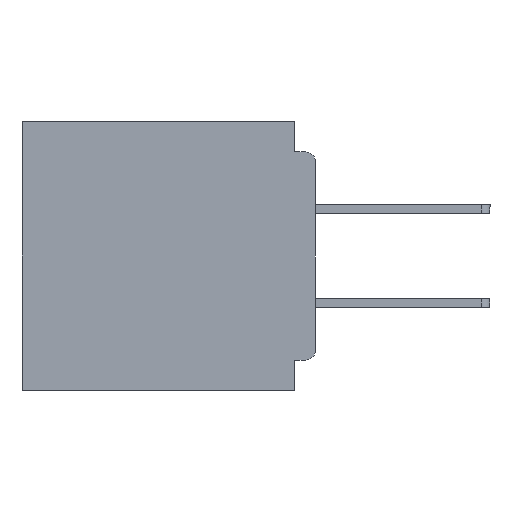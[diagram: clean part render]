
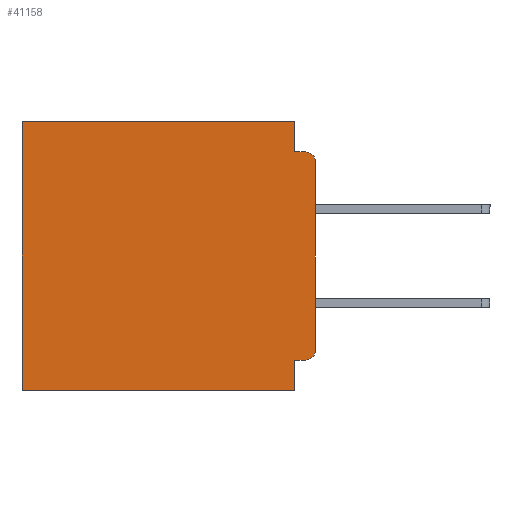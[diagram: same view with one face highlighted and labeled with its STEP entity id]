
A CAD part, left-side view. The second image highlights one B-rep face of the part: STEP entity #41158.
In plain terms, the highlighted planar face has unit normal (-1, 0, 0).
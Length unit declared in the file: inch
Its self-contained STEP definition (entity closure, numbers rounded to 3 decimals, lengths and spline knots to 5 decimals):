
#949 = EDGE_CURVE ( 'NONE', #23694, #44649, #47335, .T. ) ;
#1743 = VERTEX_POINT ( 'NONE', #13248 ) ;
#1891 = ORIENTED_EDGE ( 'NONE', *, *, #44778, .F. ) ;
#1966 = DIRECTION ( 'NONE',  ( 0., 0., -1. ) ) ;
#2060 = EDGE_CURVE ( 'NONE', #1743, #26895, #12864, .T. ) ;
#2621 = LINE ( 'NONE', #42442, #40899 ) ;
#3561 = ORIENTED_EDGE ( 'NONE', *, *, #24963, .F. ) ;
#4515 = LINE ( 'NONE', #44449, #32737 ) ;
#5194 = VECTOR ( 'NONE', #18913, 39.37008 ) ;
#5952 = CARTESIAN_POINT ( 'NONE',  ( 0.3, 0.015, -0.06 ) ) ;
#6795 = CARTESIAN_POINT ( 'NONE',  ( 0.3, 0.437, 0. ) ) ;
#7148 = LINE ( 'NONE', #17382, #15026 ) ;
#7255 = EDGE_CURVE ( 'NONE', #13311, #23694, #4515, .T. ) ;
#7734 = CARTESIAN_POINT ( 'NONE',  ( 0.3, 0.015, -0.34 ) ) ;
#9038 = VERTEX_POINT ( 'NONE', #13442 ) ;
#9049 = EDGE_CURVE ( 'NONE', #20914, #44649, #18894, .T. ) ;
#9212 = LINE ( 'NONE', #17850, #28392 ) ;
#9858 = DIRECTION ( 'NONE',  ( 0., 0., -1. ) ) ;
#9873 = AXIS2_PLACEMENT_3D ( 'NONE', #5952, #32758, #9858 ) ;
#10303 = CARTESIAN_POINT ( 'NONE',  ( 0.3, 0.015, -0.045 ) ) ;
#10361 = DIRECTION ( 'NONE',  ( 0., 0., -1. ) ) ;
#10564 = CARTESIAN_POINT ( 'NONE',  ( 0.3, 0., -0.06 ) ) ;
#10744 = DIRECTION ( 'NONE',  ( 1., 0., 0. ) ) ;
#11094 = ORIENTED_EDGE ( 'NONE', *, *, #7255, .F. ) ;
#11638 = DIRECTION ( 'NONE',  ( 0., 0., -1. ) ) ;
#11641 = VECTOR ( 'NONE', #14758, 39.37008 ) ;
#12192 = ORIENTED_EDGE ( 'NONE', *, *, #46642, .T. ) ;
#12536 = VERTEX_POINT ( 'NONE', #6795 ) ;
#12864 = LINE ( 'NONE', #44875, #11641 ) ;
#13248 = CARTESIAN_POINT ( 'NONE',  ( 0.3, 0.031, -0.355 ) ) ;
#13311 = VERTEX_POINT ( 'NONE', #25692 ) ;
#13442 = CARTESIAN_POINT ( 'NONE',  ( 0.3, 0.015, -0.355 ) ) ;
#13733 = EDGE_CURVE ( 'NONE', #12536, #34323, #7148, .T. ) ;
#14758 = DIRECTION ( 'NONE',  ( 0., 0., -1. ) ) ;
#15026 = VECTOR ( 'NONE', #1966, 39.37008 ) ;
#15034 = CARTESIAN_POINT ( 'NONE',  ( 0.3, 0., -0.355 ) ) ;
#17126 = VECTOR ( 'NONE', #33660, 39.37008 ) ;
#17382 = CARTESIAN_POINT ( 'NONE',  ( 0.3, 0.437, -0.4 ) ) ;
#17461 = LINE ( 'NONE', #19959, #38786 ) ;
#17728 = ORIENTED_EDGE ( 'NONE', *, *, #9049, .T. ) ;
#17850 = CARTESIAN_POINT ( 'NONE',  ( 0.3, 0., -0.4 ) ) ;
#18521 = CARTESIAN_POINT ( 'NONE',  ( 0.3, 0., -0.4 ) ) ;
#18894 = CIRCLE ( 'NONE', #9873, 0.015 ) ;
#18913 = DIRECTION ( 'NONE',  ( 0., 1., 0. ) ) ;
#19959 = CARTESIAN_POINT ( 'NONE',  ( 0.3, 0., -0.4 ) ) ;
#20795 = EDGE_LOOP ( 'NONE', ( #25402, #17728, #23569, #11094, #36099, #27829, #3561, #35887, #1891, #12192 ) ) ;
#20914 = VERTEX_POINT ( 'NONE', #10564 ) ;
#22131 = EDGE_CURVE ( 'NONE', #13311, #12536, #2621, .T. ) ;
#23569 = ORIENTED_EDGE ( 'NONE', *, *, #949, .F. ) ;
#23694 = VERTEX_POINT ( 'NONE', #44800 ) ;
#24091 = CARTESIAN_POINT ( 'NONE',  ( 0.3, 0.031, -0.4 ) ) ;
#24963 = EDGE_CURVE ( 'NONE', #26895, #34323, #17461, .T. ) ;
#25402 = ORIENTED_EDGE ( 'NONE', *, *, #41027, .F. ) ;
#25692 = CARTESIAN_POINT ( 'NONE',  ( 0.3, 0.031, 0. ) ) ;
#26142 = DIRECTION ( 'NONE',  ( 0., 0., -1. ) ) ;
#26178 = CARTESIAN_POINT ( 'NONE',  ( 0.3, 0., -0.045 ) ) ;
#26895 = VERTEX_POINT ( 'NONE', #24091 ) ;
#27051 = VERTEX_POINT ( 'NONE', #32874 ) ;
#27829 = ORIENTED_EDGE ( 'NONE', *, *, #13733, .T. ) ;
#28392 = VECTOR ( 'NONE', #44326, 39.37008 ) ;
#28439 = CIRCLE ( 'NONE', #49419, 0.015 ) ;
#32516 = FACE_OUTER_BOUND ( 'NONE', #20795, .T. ) ;
#32737 = VECTOR ( 'NONE', #10361, 39.37008 ) ;
#32758 = DIRECTION ( 'NONE',  ( -1., 0., 0. ) ) ;
#32874 = CARTESIAN_POINT ( 'NONE',  ( 0.3, 0., -0.34 ) ) ;
#33660 = DIRECTION ( 'NONE',  ( 0., -1., 0. ) ) ;
#34323 = VERTEX_POINT ( 'NONE', #40574 ) ;
#34466 = DIRECTION ( 'NONE',  ( -1., 0., 0. ) ) ;
#35757 = LINE ( 'NONE', #15034, #5194 ) ;
#35887 = ORIENTED_EDGE ( 'NONE', *, *, #2060, .F. ) ;
#36099 = ORIENTED_EDGE ( 'NONE', *, *, #22131, .T. ) ;
#38786 = VECTOR ( 'NONE', #42610, 39.37008 ) ;
#40574 = CARTESIAN_POINT ( 'NONE',  ( 0.3, 0.437, -0.4 ) ) ;
#40899 = VECTOR ( 'NONE', #46229, 39.37008 ) ;
#41027 = EDGE_CURVE ( 'NONE', #20914, #27051, #9212, .T. ) ;
#41158 = ADVANCED_FACE ( 'NONE', ( #32516 ), #48794, .F. ) ;
#42442 = CARTESIAN_POINT ( 'NONE',  ( 0.3, 0., 0. ) ) ;
#42610 = DIRECTION ( 'NONE',  ( 0., 1., 0. ) ) ;
#44326 = DIRECTION ( 'NONE',  ( 0., 0., -1. ) ) ;
#44449 = CARTESIAN_POINT ( 'NONE',  ( 0.3, 0.031, 0. ) ) ;
#44649 = VERTEX_POINT ( 'NONE', #10303 ) ;
#44778 = EDGE_CURVE ( 'NONE', #9038, #1743, #35757, .T. ) ;
#44800 = CARTESIAN_POINT ( 'NONE',  ( 0.3, 0.031, -0.045 ) ) ;
#44875 = CARTESIAN_POINT ( 'NONE',  ( 0.3, 0.031, -0.4 ) ) ;
#46229 = DIRECTION ( 'NONE',  ( 0., 1., 0. ) ) ;
#46363 = AXIS2_PLACEMENT_3D ( 'NONE', #18521, #10744, #26142 ) ;
#46642 = EDGE_CURVE ( 'NONE', #9038, #27051, #28439, .T. ) ;
#47335 = LINE ( 'NONE', #26178, #17126 ) ;
#48794 = PLANE ( 'NONE',  #46363 ) ;
#49419 = AXIS2_PLACEMENT_3D ( 'NONE', #7734, #34466, #11638 ) ;
